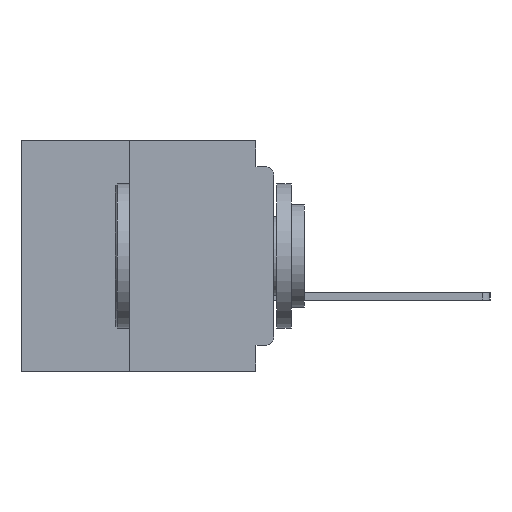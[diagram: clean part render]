
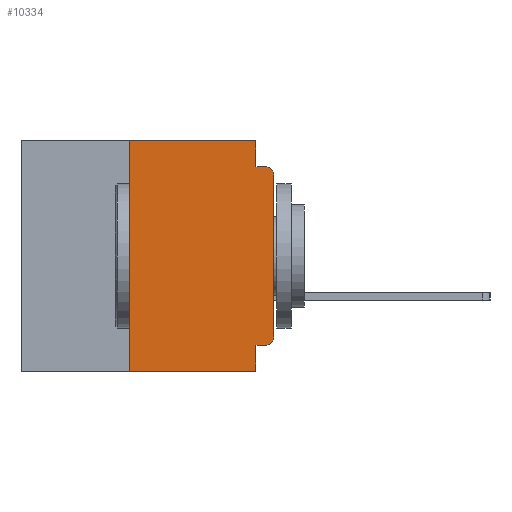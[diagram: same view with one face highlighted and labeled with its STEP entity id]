
A CAD part, left-side view. The second image highlights one B-rep face of the part: STEP entity #10334.
In plain terms, the highlighted planar face has unit normal (-1, 0, 0).
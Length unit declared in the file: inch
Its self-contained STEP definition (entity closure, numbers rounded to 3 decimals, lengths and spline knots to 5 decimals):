
#148 = EDGE_LOOP ( 'NONE', ( #8324, #1416, #18872, #21664, #8802, #5588, #21225, #31773, #17073, #19855 ) ) ;
#354 = CARTESIAN_POINT ( 'NONE',  ( 0., 0.437, -0.4 ) ) ;
#568 = FACE_OUTER_BOUND ( 'NONE', #148, .T. ) ;
#583 = CARTESIAN_POINT ( 'NONE',  ( 0., 0.015, -0.045 ) ) ;
#1416 = ORIENTED_EDGE ( 'NONE', *, *, #7908, .T. ) ;
#1423 = CARTESIAN_POINT ( 'NONE',  ( 0., 0.015, -0.06 ) ) ;
#2565 = EDGE_CURVE ( 'NONE', #16435, #5742, #20435, .T. ) ;
#2902 = DIRECTION ( 'NONE',  ( 0., 1., 0. ) ) ;
#3328 = DIRECTION ( 'NONE',  ( 0., -1., 0. ) ) ;
#3560 = CARTESIAN_POINT ( 'NONE',  ( 0., 0.25, -0.4 ) ) ;
#4226 = DIRECTION ( 'NONE',  ( 0., -1., 0. ) ) ;
#4377 = DIRECTION ( 'NONE',  ( 0., 0., -1. ) ) ;
#4710 = DIRECTION ( 'NONE',  ( 0., -1., 0. ) ) ;
#4746 = AXIS2_PLACEMENT_3D ( 'NONE', #1423, #21987, #4377 ) ;
#4868 = LINE ( 'NONE', #7820, #27394 ) ;
#5158 = EDGE_CURVE ( 'NONE', #14617, #21779, #18341, .T. ) ;
#5588 = ORIENTED_EDGE ( 'NONE', *, *, #33629, .F. ) ;
#5742 = VERTEX_POINT ( 'NONE', #11995 ) ;
#6350 = LINE ( 'NONE', #10485, #35677 ) ;
#6748 = CARTESIAN_POINT ( 'NONE',  ( 0., 0.015, -0.355 ) ) ;
#6832 = DIRECTION ( 'NONE',  ( 0., 0., -1. ) ) ;
#6864 = DIRECTION ( 'NONE',  ( -1., 0., 0. ) ) ;
#6914 = CARTESIAN_POINT ( 'NONE',  ( 0., 0.015, -0.34 ) ) ;
#7578 = CARTESIAN_POINT ( 'NONE',  ( 0., 0.031, -0.4 ) ) ;
#7820 = CARTESIAN_POINT ( 'NONE',  ( 0., 0., 0. ) ) ;
#7908 = EDGE_CURVE ( 'NONE', #24652, #25699, #9444, .T. ) ;
#8013 = AXIS2_PLACEMENT_3D ( 'NONE', #18199, #35867, #18316 ) ;
#8324 = ORIENTED_EDGE ( 'NONE', *, *, #17291, .T. ) ;
#8802 = ORIENTED_EDGE ( 'NONE', *, *, #30684, .F. ) ;
#9053 = VERTEX_POINT ( 'NONE', #12002 ) ;
#9444 = CIRCLE ( 'NONE', #4746, 0.015 ) ;
#10135 = CARTESIAN_POINT ( 'NONE',  ( 0., 0.437, 0. ) ) ;
#10334 = ADVANCED_FACE ( 'NONE', ( #568 ), #15397, .F. ) ;
#10485 = CARTESIAN_POINT ( 'NONE',  ( 0., 0., -0.045 ) ) ;
#10520 = DIRECTION ( 'NONE',  ( 0., 0., -1. ) ) ;
#11995 = CARTESIAN_POINT ( 'NONE',  ( 0., 0., -0.34 ) ) ;
#12002 = CARTESIAN_POINT ( 'NONE',  ( 0., 0.031, 0. ) ) ;
#12466 = VERTEX_POINT ( 'NONE', #31988 ) ;
#12484 = CARTESIAN_POINT ( 'NONE',  ( 0., 0.25, 0. ) ) ;
#13843 = LINE ( 'NONE', #3560, #36299 ) ;
#14617 = VERTEX_POINT ( 'NONE', #27158 ) ;
#15330 = VECTOR ( 'NONE', #10520, 39.37008 ) ;
#15397 = PLANE ( 'NONE',  #8013 ) ;
#16236 = VECTOR ( 'NONE', #18890, 39.37008 ) ;
#16435 = VERTEX_POINT ( 'NONE', #6748 ) ;
#17073 = ORIENTED_EDGE ( 'NONE', *, *, #29680, .F. ) ;
#17291 = EDGE_CURVE ( 'NONE', #5742, #24652, #4868, .T. ) ;
#17495 = VECTOR ( 'NONE', #2902, 39.37008 ) ;
#18199 = CARTESIAN_POINT ( 'NONE',  ( 0., 0.437, 0. ) ) ;
#18283 = DIRECTION ( 'NONE',  ( 0., 0., 1. ) ) ;
#18316 = DIRECTION ( 'NONE',  ( 0., 0., -1. ) ) ;
#18341 = LINE ( 'NONE', #354, #33024 ) ;
#18612 = VECTOR ( 'NONE', #4226, 39.37008 ) ;
#18872 = ORIENTED_EDGE ( 'NONE', *, *, #25304, .F. ) ;
#18890 = DIRECTION ( 'NONE',  ( 0., 0., -1. ) ) ;
#18993 = LINE ( 'NONE', #33380, #16236 ) ;
#19855 = ORIENTED_EDGE ( 'NONE', *, *, #2565, .T. ) ;
#20435 = CIRCLE ( 'NONE', #35793, 0.015 ) ;
#20751 = EDGE_CURVE ( 'NONE', #9053, #30680, #18993, .T. ) ;
#21225 = ORIENTED_EDGE ( 'NONE', *, *, #5158, .T. ) ;
#21664 = ORIENTED_EDGE ( 'NONE', *, *, #20751, .F. ) ;
#21779 = VERTEX_POINT ( 'NONE', #26290 ) ;
#21987 = DIRECTION ( 'NONE',  ( -1., 0., 0. ) ) ;
#24652 = VERTEX_POINT ( 'NONE', #31076 ) ;
#24780 = CARTESIAN_POINT ( 'NONE',  ( 0., 0.031, -0.045 ) ) ;
#25304 = EDGE_CURVE ( 'NONE', #30680, #25699, #6350, .T. ) ;
#25319 = LINE ( 'NONE', #34933, #17495 ) ;
#25699 = VERTEX_POINT ( 'NONE', #583 ) ;
#26290 = CARTESIAN_POINT ( 'NONE',  ( 0., 0.031, -0.4 ) ) ;
#26447 = LINE ( 'NONE', #10135, #18612 ) ;
#26573 = VERTEX_POINT ( 'NONE', #12484 ) ;
#27158 = CARTESIAN_POINT ( 'NONE',  ( 0., 0.25, -0.4 ) ) ;
#27394 = VECTOR ( 'NONE', #37138, 39.37008 ) ;
#29680 = EDGE_CURVE ( 'NONE', #16435, #12466, #25319, .T. ) ;
#30680 = VERTEX_POINT ( 'NONE', #24780 ) ;
#30684 = EDGE_CURVE ( 'NONE', #26573, #9053, #26447, .T. ) ;
#31076 = CARTESIAN_POINT ( 'NONE',  ( 0., 0., -0.06 ) ) ;
#31773 = ORIENTED_EDGE ( 'NONE', *, *, #32547, .F. ) ;
#31988 = CARTESIAN_POINT ( 'NONE',  ( 0., 0.031, -0.355 ) ) ;
#32547 = EDGE_CURVE ( 'NONE', #12466, #21779, #37740, .T. ) ;
#33024 = VECTOR ( 'NONE', #3328, 39.37008 ) ;
#33380 = CARTESIAN_POINT ( 'NONE',  ( 0., 0.031, 0. ) ) ;
#33629 = EDGE_CURVE ( 'NONE', #14617, #26573, #13843, .T. ) ;
#34933 = CARTESIAN_POINT ( 'NONE',  ( 0., 0., -0.355 ) ) ;
#35677 = VECTOR ( 'NONE', #4710, 39.37008 ) ;
#35793 = AXIS2_PLACEMENT_3D ( 'NONE', #6914, #6864, #6832 ) ;
#35867 = DIRECTION ( 'NONE',  ( 1., 0., 0. ) ) ;
#36299 = VECTOR ( 'NONE', #18283, 39.37008 ) ;
#37138 = DIRECTION ( 'NONE',  ( 0., 0., 1. ) ) ;
#37740 = LINE ( 'NONE', #7578, #15330 ) ;
